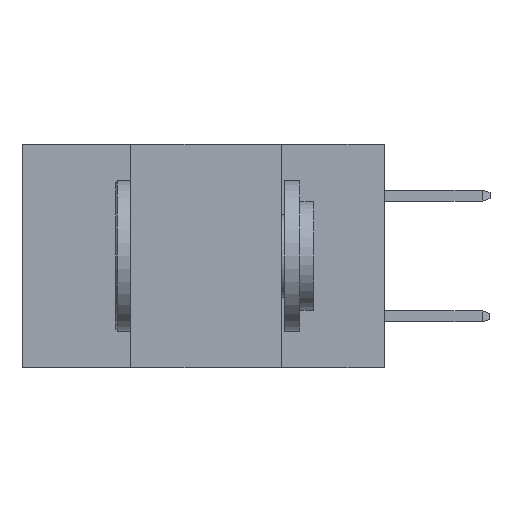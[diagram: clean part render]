
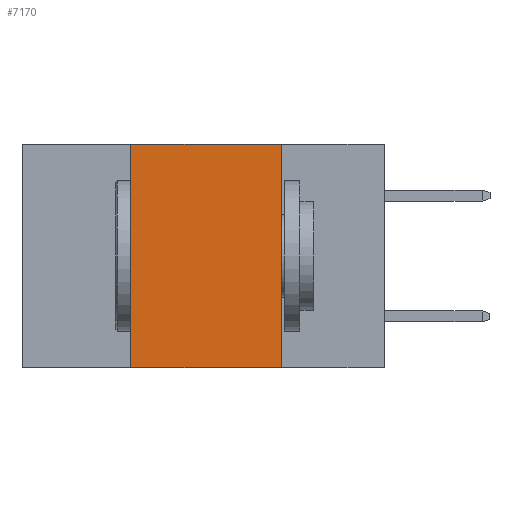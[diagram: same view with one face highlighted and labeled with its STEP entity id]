
A CAD part, left-side view. The second image highlights one B-rep face of the part: STEP entity #7170.
In plain terms, the highlighted planar face has unit normal (-1, 0, 0).
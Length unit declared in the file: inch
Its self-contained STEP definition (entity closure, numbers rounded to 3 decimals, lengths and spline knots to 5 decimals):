
#241 = ORIENTED_EDGE ( 'NONE', *, *, #16507, .F. ) ;
#418 = EDGE_CURVE ( 'NONE', #988, #8577, #4041, .T. ) ;
#988 = VERTEX_POINT ( 'NONE', #4701 ) ;
#2173 = CARTESIAN_POINT ( 'NONE',  ( 0., 0.42, -0.37 ) ) ;
#4012 = LINE ( 'NONE', #14645, #15652 ) ;
#4016 = CARTESIAN_POINT ( 'NONE',  ( 0., 0.6, 0. ) ) ;
#4041 = LINE ( 'NONE', #17461, #16166 ) ;
#4268 = ORIENTED_EDGE ( 'NONE', *, *, #418, .F. ) ;
#4664 = CARTESIAN_POINT ( 'NONE',  ( 0., 0.17, 0. ) ) ;
#4701 = CARTESIAN_POINT ( 'NONE',  ( 0., 0.42, 0. ) ) ;
#5648 = DIRECTION ( 'NONE',  ( 1., 0., 0. ) ) ;
#6269 = DIRECTION ( 'NONE',  ( 0., 0., -1. ) ) ;
#6506 = LINE ( 'NONE', #4664, #18585 ) ;
#6593 = VECTOR ( 'NONE', #18630, 39.37008 ) ;
#7170 = ADVANCED_FACE ( 'NONE', ( #17547 ), #10305, .F. ) ;
#8577 = VERTEX_POINT ( 'NONE', #13887 ) ;
#10305 = PLANE ( 'NONE',  #16234 ) ;
#10795 = LINE ( 'NONE', #13894, #6593 ) ;
#12225 = ORIENTED_EDGE ( 'NONE', *, *, #17565, .F. ) ;
#13069 = CARTESIAN_POINT ( 'NONE',  ( 0., 0.17, -0.37 ) ) ;
#13887 = CARTESIAN_POINT ( 'NONE',  ( 0., 0.17, 0. ) ) ;
#13894 = CARTESIAN_POINT ( 'NONE',  ( 0., 0.6, -0.37 ) ) ;
#14409 = EDGE_CURVE ( 'NONE', #14859, #16489, #10795, .T. ) ;
#14645 = CARTESIAN_POINT ( 'NONE',  ( 0., 0.42, 0. ) ) ;
#14694 = ORIENTED_EDGE ( 'NONE', *, *, #14409, .T. ) ;
#14859 = VERTEX_POINT ( 'NONE', #2173 ) ;
#15652 = VECTOR ( 'NONE', #16228, 39.37008 ) ;
#16166 = VECTOR ( 'NONE', #18704, 39.37008 ) ;
#16228 = DIRECTION ( 'NONE',  ( 0., 0., 1. ) ) ;
#16234 = AXIS2_PLACEMENT_3D ( 'NONE', #4016, #5648, #16671 ) ;
#16489 = VERTEX_POINT ( 'NONE', #13069 ) ;
#16507 = EDGE_CURVE ( 'NONE', #14859, #988, #4012, .T. ) ;
#16671 = DIRECTION ( 'NONE',  ( 0., 0., -1. ) ) ;
#17461 = CARTESIAN_POINT ( 'NONE',  ( 0., 0.6, 0. ) ) ;
#17547 = FACE_OUTER_BOUND ( 'NONE', #19028, .T. ) ;
#17565 = EDGE_CURVE ( 'NONE', #8577, #16489, #6506, .T. ) ;
#18585 = VECTOR ( 'NONE', #6269, 39.37008 ) ;
#18630 = DIRECTION ( 'NONE',  ( 0., -1., 0. ) ) ;
#18704 = DIRECTION ( 'NONE',  ( 0., -1., 0. ) ) ;
#19028 = EDGE_LOOP ( 'NONE', ( #12225, #4268, #241, #14694 ) ) ;
